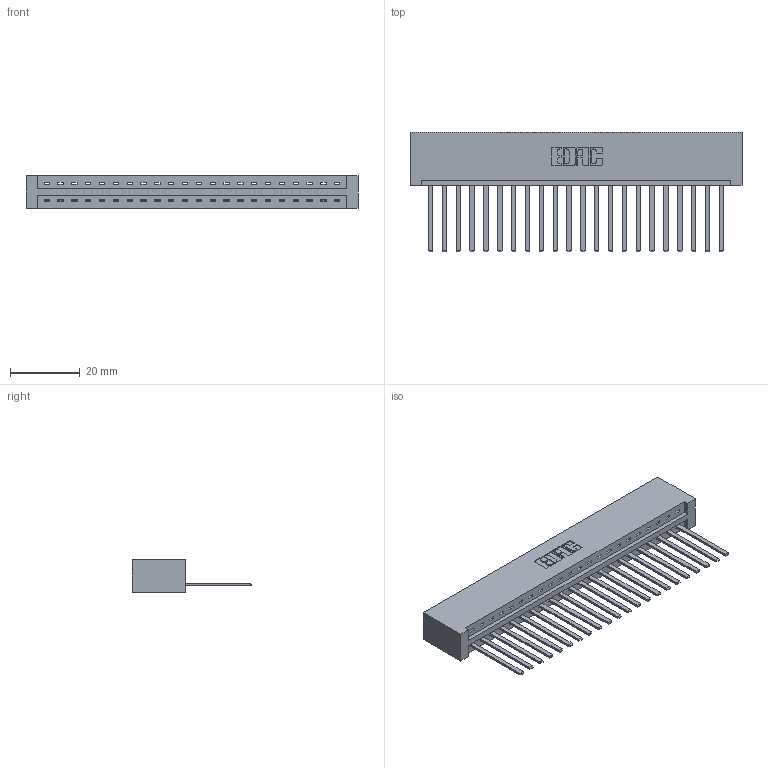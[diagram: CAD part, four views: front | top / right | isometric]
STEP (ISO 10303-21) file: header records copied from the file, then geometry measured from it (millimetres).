
FILE_DESCRIPTION (( 'STEP AP203' ), '1' );
FILE_NAME ('337-022-544-101.STEP', '2018-08-05T14:41:40', ( '' ), ( '' ), 'SwSTEP 2.0', 'SolidWorks 2016', '' );
FILE_SCHEMA (( 'CONFIG_CONTROL_DESIGN' ));
Length unit declared in the file: inch
Products named in the file (3): 337-022-544-101; 337 Part_No Mounting Lugs; 345-292-001_345-293-144
Assembly tree (23 placements, depth 2):
  337-022-544-101
    337 Part_No Mounting Lugs
    345-292-001_345-293-144  x22
Bounding box: 95.05 x 34.3 x 9.4 mm (x, y, z)
Volume: 10621.7 mm3; surface area: 11684.6 mm2
Topology: 23 solids, 23 shells, 1338 faces, 4027 edges, 2654 vertices
Faces by surface type: plane 990, cylinder 348
Entity records: 18479 total; most frequent: CARTESIAN_POINT 3224, ORIENTED_EDGE 3182, DIRECTION 2743, EDGE_CURVE 1591, LINE 1475, VECTOR 1475, VERTEX_POINT 1058, AXIS2_PLACEMENT_3D 634
